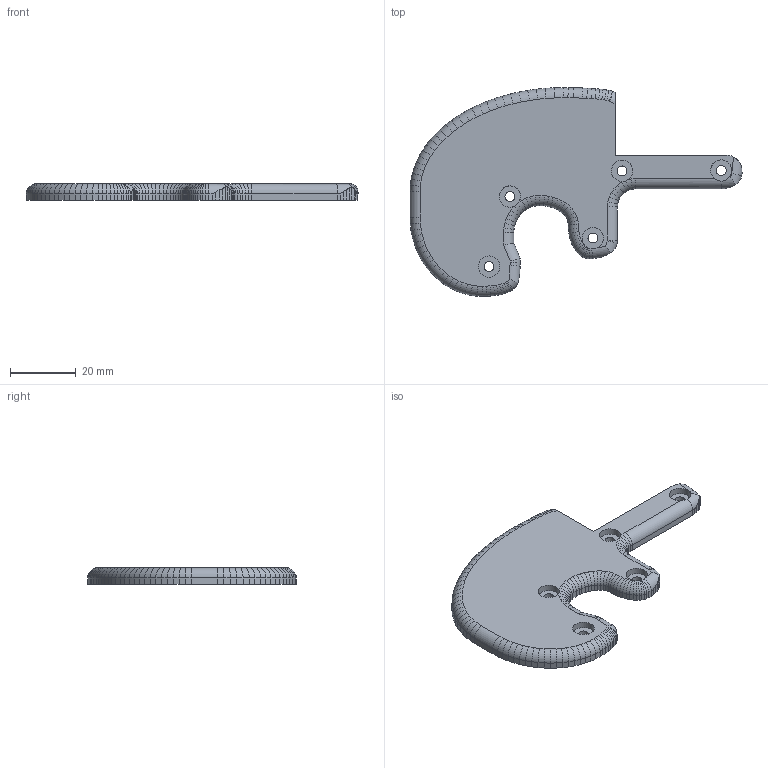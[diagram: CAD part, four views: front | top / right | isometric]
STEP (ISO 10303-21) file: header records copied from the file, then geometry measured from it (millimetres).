
FILE_DESCRIPTION((''),'2;1');
FILE_NAME('derringer-RR.stp','2013-07-11T16:53:32',('mrfr'),(''),'Autodesk Inventor 2013','Autodesk Inventor 2013','');
FILE_SCHEMA(('AUTOMOTIVE_DESIGN { 1 0 10303 214 1 1 1 1 }'));
Length unit declared in the file: millimetre
Products named in the file (1): derringer-RR
Bounding box: 101.33 x 63.76 x 5 mm (x, y, z)
Volume: 15793.4 mm3; surface area: 8203.1 mm2
Topology: 1 solids, 1 shells, 307 faces, 785 edges, 481 vertices
Faces by surface type: plane 165, cylinder 142
Full cylindrical faces by diameter (mm): 3 x5, 6.5 x5
Entity records: 9139 total; most frequent: CARTESIAN_POINT 1670, DIRECTION 1545, ORIENTED_EDGE 1542, EDGE_CURVE 771, VECTOR 581, LINE 581, AXIS2_PLACEMENT_3D 482, VERTEX_POINT 477
